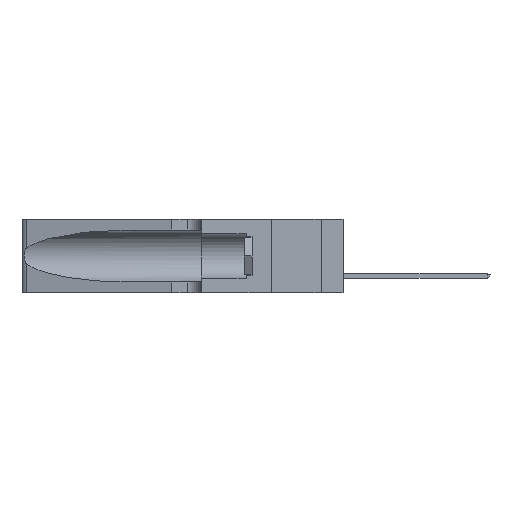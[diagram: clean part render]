
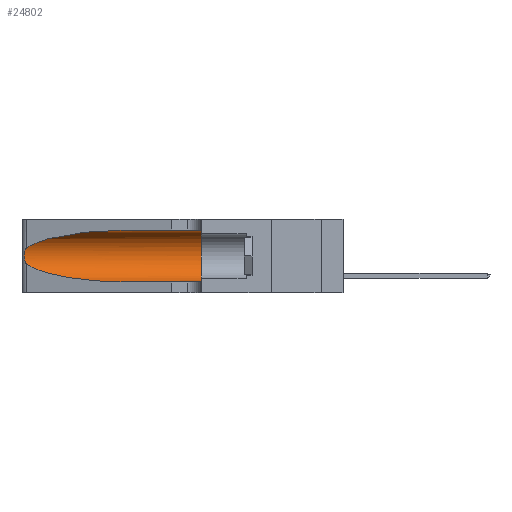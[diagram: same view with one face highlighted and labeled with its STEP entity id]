
A CAD part, left-side view. The second image highlights one B-rep face of the part: STEP entity #24802.
In plain terms, the highlighted cylindrical face has radius 3.308 mm (diameter 6.617 mm), a partial arc.
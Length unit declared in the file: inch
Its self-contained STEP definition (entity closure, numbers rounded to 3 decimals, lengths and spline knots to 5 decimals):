
#1394 = CARTESIAN_POINT ( 'NONE',  ( 0.26017, 1.23833, 0.17102 ) ) ;
#1556 = CARTESIAN_POINT ( 'NONE',  ( 0.25787, 1.23484, 0.2124 ) ) ;
#1596 = CARTESIAN_POINT ( 'NONE',  ( 0.1305, 0.35, 0.185 ) ) ;
#1717 = CARTESIAN_POINT ( 'NONE',  ( 0.26018, 1.23835, 0.19895 ) ) ;
#1886 = CARTESIAN_POINT ( 'NONE',  ( 0.25789, 1.23486, 0.15765 ) ) ;
#2064 = FACE_OUTER_BOUND ( 'NONE', #42000, .T. ) ;
#2324 = CARTESIAN_POINT ( 'NONE',  ( 0.1305, 1.61858, 0.05475 ) ) ;
#3202 = ORIENTED_EDGE ( 'NONE', *, *, #12393, .T. ) ;
#4765 = CARTESIAN_POINT ( 'NONE',  ( 0.26075, 1.23896, 0.178 ) ) ;
#5339 = ORIENTED_EDGE ( 'NONE', *, *, #17991, .F. ) ;
#5646 = ORIENTED_EDGE ( 'NONE', *, *, #39781, .T. ) ;
#7994 = CARTESIAN_POINT ( 'NONE',  ( 0.25555, 1.22994, 0.2215 ) ) ;
#8489 = CARTESIAN_POINT ( 'NONE',  ( 0.25856, 1.23593, 0.16098 ) ) ;
#8524 = DIRECTION ( 'NONE',  ( 0., 1., 0. ) ) ;
#9344 = CARTESIAN_POINT ( 'NONE',  ( 0.1305, 0.35, 0.05475 ) ) ;
#10045 = VERTEX_POINT ( 'NONE', #9344 ) ;
#10251 = ORIENTED_EDGE ( 'NONE', *, *, #25971, .F. ) ;
#12393 = EDGE_CURVE ( 'NONE', #35456, #37774, #20218, .T. ) ;
#12714 = VERTEX_POINT ( 'NONE', #32151 ) ;
#12821 = CARTESIAN_POINT ( 'NONE',  ( 0.1305, 0.72297, 0.31525 ) ) ;
#13984 = CARTESIAN_POINT ( 'NONE',  ( 0.25487, 1.22718, 0.14631 ) ) ;
#14938 = CARTESIAN_POINT ( 'NONE',  ( 0.25555, 1.22993, 0.14849 ) ) ;
#16389 = ORIENTED_EDGE ( 'NONE', *, *, #24622, .T. ) ;
#17991 = EDGE_CURVE ( 'NONE', #26191, #43208, #31500, .T. ) ;
#18115 = DIRECTION ( 'NONE',  ( 0., -1., 0. ) ) ;
#18875 =( BOUNDED_CURVE ( )  B_SPLINE_CURVE ( 3, ( #29174, #39341, #37105, #40184 ),
 .UNSPECIFIED., .F., .F. ) 
 B_SPLINE_CURVE_WITH_KNOTS ( ( 4, 4 ),
 ( 3.44316, 4.71239 ),
 .UNSPECIFIED. ) 
 CURVE ( )  GEOMETRIC_REPRESENTATION_ITEM ( )  RATIONAL_B_SPLINE_CURVE ( ( 1., 0.87, 0.87, 1. ) ) 
 REPRESENTATION_ITEM ( '' )  );
#19131 = DIRECTION ( 'NONE',  ( 0., -1., 0. ) ) ;
#20218 = B_SPLINE_CURVE_WITH_KNOTS ( 'NONE', 3,
 ( #38828, #7994, #31721, #1556, #35594, #1717, #25391, #4765, #1394, #8489, #1886, #25545, #14938, #31884 ),
 .UNSPECIFIED., .F., .F.,
 ( 4, 2, 2, 2, 2, 2, 4 ),
 ( 0., 0.00027, 0.00053, 0.00107, 0.0016, 0.00187, 0.00214 ),
 .UNSPECIFIED. ) ;
#20395 = CIRCLE ( 'NONE', #27199, 0.13025 ) ;
#20992 = CYLINDRICAL_SURFACE ( 'NONE', #36525, 0.13025 ) ;
#22975 =( BOUNDED_CURVE ( )  B_SPLINE_CURVE ( 3, ( #41840, #26559, #26115, #43072 ),
 .UNSPECIFIED., .F., .F. ) 
 B_SPLINE_CURVE_WITH_KNOTS ( ( 4, 4 ),
 ( 1.5708, 2.84003 ),
 .UNSPECIFIED. ) 
 CURVE ( )  GEOMETRIC_REPRESENTATION_ITEM ( )  RATIONAL_B_SPLINE_CURVE ( ( 1., 0.87, 0.87, 1. ) ) 
 REPRESENTATION_ITEM ( '' )  );
#24622 = EDGE_CURVE ( 'NONE', #12714, #10045, #29091, .T. ) ;
#24752 = VECTOR ( 'NONE', #19131, 39.37008 ) ;
#24802 = ADVANCED_FACE ( 'NONE', ( #2064 ), #20992, .F. ) ;
#25391 = CARTESIAN_POINT ( 'NONE',  ( 0.26075, 1.23896, 0.19203 ) ) ;
#25545 = CARTESIAN_POINT ( 'NONE',  ( 0.25639, 1.23186, 0.15144 ) ) ;
#25971 = EDGE_CURVE ( 'NONE', #43208, #10045, #20395, .T. ) ;
#26115 = CARTESIAN_POINT ( 'NONE',  ( 0.2373, 1.15595, 0.28018 ) ) ;
#26191 = VERTEX_POINT ( 'NONE', #12821 ) ;
#26217 = EDGE_CURVE ( 'NONE', #37774, #12714, #18875, .T. ) ;
#26559 = CARTESIAN_POINT ( 'NONE',  ( 0.18966, 0.96281, 0.31525 ) ) ;
#27199 = AXIS2_PLACEMENT_3D ( 'NONE', #1596, #8524, #39594 ) ;
#27210 = CARTESIAN_POINT ( 'NONE',  ( 0.1305, 0.35, 0.31525 ) ) ;
#27825 = VECTOR ( 'NONE', #39805, 39.37008 ) ;
#28579 = CARTESIAN_POINT ( 'NONE',  ( 0.25487, 1.22718, 0.22369 ) ) ;
#29091 = LINE ( 'NONE', #2324, #24752 ) ;
#29174 = CARTESIAN_POINT ( 'NONE',  ( 0.25487, 1.22718, 0.14631 ) ) ;
#31500 = LINE ( 'NONE', #40088, #27825 ) ;
#31721 = CARTESIAN_POINT ( 'NONE',  ( 0.25639, 1.23184, 0.21858 ) ) ;
#31884 = CARTESIAN_POINT ( 'NONE',  ( 0.25487, 1.22718, 0.14631 ) ) ;
#32151 = CARTESIAN_POINT ( 'NONE',  ( 0.1305, 0.72297, 0.05475 ) ) ;
#35014 = CARTESIAN_POINT ( 'NONE',  ( 0.1305, 1.61858, 0.185 ) ) ;
#35456 = VERTEX_POINT ( 'NONE', #28579 ) ;
#35594 = CARTESIAN_POINT ( 'NONE',  ( 0.25854, 1.2359, 0.20912 ) ) ;
#36525 = AXIS2_PLACEMENT_3D ( 'NONE', #35014, #18115, #41749 ) ;
#37105 = CARTESIAN_POINT ( 'NONE',  ( 0.18966, 0.96281, 0.05475 ) ) ;
#37774 = VERTEX_POINT ( 'NONE', #13984 ) ;
#38828 = CARTESIAN_POINT ( 'NONE',  ( 0.25487, 1.22718, 0.22369 ) ) ;
#39341 = CARTESIAN_POINT ( 'NONE',  ( 0.2373, 1.15595, 0.08982 ) ) ;
#39594 = DIRECTION ( 'NONE',  ( 0., 0., 1. ) ) ;
#39781 = EDGE_CURVE ( 'NONE', #26191, #35456, #22975, .T. ) ;
#39805 = DIRECTION ( 'NONE',  ( 0., -1., 0. ) ) ;
#40088 = CARTESIAN_POINT ( 'NONE',  ( 0.1305, 1.61858, 0.31525 ) ) ;
#40184 = CARTESIAN_POINT ( 'NONE',  ( 0.1305, 0.72297, 0.05475 ) ) ;
#41252 = ORIENTED_EDGE ( 'NONE', *, *, #26217, .T. ) ;
#41749 = DIRECTION ( 'NONE',  ( 0., 0., -1. ) ) ;
#41840 = CARTESIAN_POINT ( 'NONE',  ( 0.1305, 0.72297, 0.31525 ) ) ;
#42000 = EDGE_LOOP ( 'NONE', ( #5646, #3202, #41252, #16389, #10251, #5339 ) ) ;
#43072 = CARTESIAN_POINT ( 'NONE',  ( 0.25487, 1.22718, 0.22369 ) ) ;
#43208 = VERTEX_POINT ( 'NONE', #27210 ) ;
